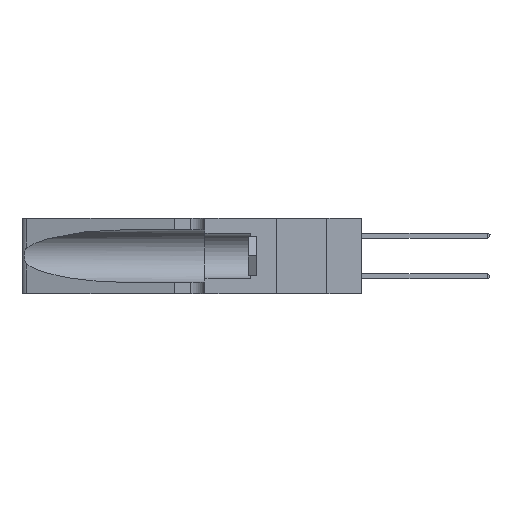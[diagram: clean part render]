
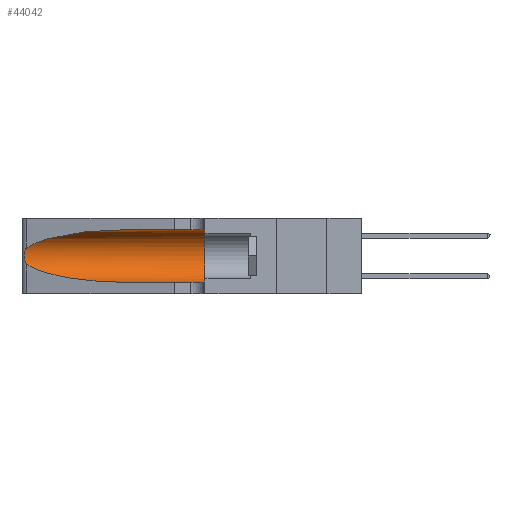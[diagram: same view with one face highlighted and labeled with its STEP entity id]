
A CAD part, left-side view. The second image highlights one B-rep face of the part: STEP entity #44042.
In plain terms, the highlighted cylindrical face has radius 3.308 mm (diameter 6.617 mm), a partial arc.
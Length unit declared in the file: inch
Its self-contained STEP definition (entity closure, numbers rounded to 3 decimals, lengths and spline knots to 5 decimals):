
#863 = CARTESIAN_POINT ( 'NONE',  ( 0.25854, 1.2359, 0.20912 ) ) ;
#1020 = CARTESIAN_POINT ( 'NONE',  ( 0.26018, 1.23835, 0.19895 ) ) ;
#1351 = DIRECTION ( 'NONE',  ( 0., -1., 0. ) ) ;
#1373 = VERTEX_POINT ( 'NONE', #34866 ) ;
#1954 = VERTEX_POINT ( 'NONE', #18898 ) ;
#2078 = DIRECTION ( 'NONE',  ( 0., -1., 0. ) ) ;
#2092 = AXIS2_PLACEMENT_3D ( 'NONE', #46518, #17487, #35357 ) ;
#2731 = CARTESIAN_POINT ( 'NONE',  ( 0.1305, 0.72297, 0.31525 ) ) ;
#3497 = CARTESIAN_POINT ( 'NONE',  ( 0.18966, 0.96281, 0.31525 ) ) ;
#3887 = ORIENTED_EDGE ( 'NONE', *, *, #15033, .T. ) ;
#4369 = CARTESIAN_POINT ( 'NONE',  ( 0.26075, 1.23896, 0.178 ) ) ;
#4590 = DIRECTION ( 'NONE',  ( 0., -1., 0. ) ) ;
#4843 = CARTESIAN_POINT ( 'NONE',  ( 0.25555, 1.22993, 0.14849 ) ) ;
#4985 = EDGE_CURVE ( 'NONE', #29005, #1954, #27852, .T. ) ;
#5172 = CARTESIAN_POINT ( 'NONE',  ( 0.1305, 1.61858, 0.185 ) ) ;
#7144 = CARTESIAN_POINT ( 'NONE',  ( 0.1305, 0.72297, 0.31525 ) ) ;
#7342 = AXIS2_PLACEMENT_3D ( 'NONE', #5172, #1351, #18997 ) ;
#7555 =( BOUNDED_CURVE ( )  B_SPLINE_CURVE ( 3, ( #23868, #20100, #12481, #26851 ),
 .UNSPECIFIED., .F., .F. ) 
 B_SPLINE_CURVE_WITH_KNOTS ( ( 4, 4 ),
 ( 3.44316, 4.71239 ),
 .UNSPECIFIED. ) 
 CURVE ( )  GEOMETRIC_REPRESENTATION_ITEM ( )  RATIONAL_B_SPLINE_CURVE ( ( 1., 0.87, 0.87, 1. ) ) 
 REPRESENTATION_ITEM ( '' )  );
#8351 = CARTESIAN_POINT ( 'NONE',  ( 0.25639, 1.23184, 0.21858 ) ) ;
#11143 = CARTESIAN_POINT ( 'NONE',  ( 0.25487, 1.22718, 0.14631 ) ) ;
#11994 = ORIENTED_EDGE ( 'NONE', *, *, #39823, .T. ) ;
#12154 = CARTESIAN_POINT ( 'NONE',  ( 0.26017, 1.23833, 0.17102 ) ) ;
#12481 = CARTESIAN_POINT ( 'NONE',  ( 0.18966, 0.96281, 0.05475 ) ) ;
#15033 = EDGE_CURVE ( 'NONE', #1954, #36051, #39171, .T. ) ;
#15307 = CARTESIAN_POINT ( 'NONE',  ( 0.25487, 1.22718, 0.22369 ) ) ;
#15538 = LINE ( 'NONE', #40557, #36487 ) ;
#16273 = CYLINDRICAL_SURFACE ( 'NONE', #7342, 0.13025 ) ;
#17487 = DIRECTION ( 'NONE',  ( 0., 1., 0. ) ) ;
#18898 = CARTESIAN_POINT ( 'NONE',  ( 0.25487, 1.22718, 0.22369 ) ) ;
#18995 = CARTESIAN_POINT ( 'NONE',  ( 0.25787, 1.23484, 0.2124 ) ) ;
#18997 = DIRECTION ( 'NONE',  ( 0., 0., -1. ) ) ;
#20015 = ORIENTED_EDGE ( 'NONE', *, *, #22002, .F. ) ;
#20100 = CARTESIAN_POINT ( 'NONE',  ( 0.2373, 1.15595, 0.08982 ) ) ;
#20306 = CARTESIAN_POINT ( 'NONE',  ( 0.1305, 0.35, 0.31525 ) ) ;
#22002 = EDGE_CURVE ( 'NONE', #40436, #1373, #23542, .T. ) ;
#22773 = EDGE_CURVE ( 'NONE', #29005, #40436, #15538, .T. ) ;
#23542 = CIRCLE ( 'NONE', #2092, 0.13025 ) ;
#23868 = CARTESIAN_POINT ( 'NONE',  ( 0.25487, 1.22718, 0.14631 ) ) ;
#24752 = FACE_OUTER_BOUND ( 'NONE', #34315, .T. ) ;
#25524 = EDGE_CURVE ( 'NONE', #36051, #34071, #7555, .T. ) ;
#26526 = CARTESIAN_POINT ( 'NONE',  ( 0.25856, 1.23593, 0.16098 ) ) ;
#26631 = ORIENTED_EDGE ( 'NONE', *, *, #25524, .T. ) ;
#26851 = CARTESIAN_POINT ( 'NONE',  ( 0.1305, 0.72297, 0.05475 ) ) ;
#27852 =( BOUNDED_CURVE ( )  B_SPLINE_CURVE ( 3, ( #7144, #3497, #28830, #39300 ),
 .UNSPECIFIED., .F., .T. ) 
 B_SPLINE_CURVE_WITH_KNOTS ( ( 4, 4 ),
 ( 1.5708, 2.84003 ),
 .UNSPECIFIED. ) 
 CURVE ( )  GEOMETRIC_REPRESENTATION_ITEM ( )  RATIONAL_B_SPLINE_CURVE ( ( 1., 0.87, 0.87, 1. ) ) 
 REPRESENTATION_ITEM ( '' )  );
#28830 = CARTESIAN_POINT ( 'NONE',  ( 0.2373, 1.15595, 0.28018 ) ) ;
#29005 = VERTEX_POINT ( 'NONE', #2731 ) ;
#29709 = CARTESIAN_POINT ( 'NONE',  ( 0.25639, 1.23186, 0.15144 ) ) ;
#30171 = CARTESIAN_POINT ( 'NONE',  ( 0.25487, 1.22718, 0.14631 ) ) ;
#33665 = CARTESIAN_POINT ( 'NONE',  ( 0.26075, 1.23896, 0.19203 ) ) ;
#33702 = LINE ( 'NONE', #38201, #42814 ) ;
#34071 = VERTEX_POINT ( 'NONE', #41200 ) ;
#34315 = EDGE_LOOP ( 'NONE', ( #35476, #3887, #26631, #11994, #20015, #35733 ) ) ;
#34866 = CARTESIAN_POINT ( 'NONE',  ( 0.1305, 0.35, 0.05475 ) ) ;
#35357 = DIRECTION ( 'NONE',  ( 0., 0., 1. ) ) ;
#35476 = ORIENTED_EDGE ( 'NONE', *, *, #4985, .T. ) ;
#35733 = ORIENTED_EDGE ( 'NONE', *, *, #22773, .F. ) ;
#36051 = VERTEX_POINT ( 'NONE', #11143 ) ;
#36487 = VECTOR ( 'NONE', #4590, 39.37008 ) ;
#38201 = CARTESIAN_POINT ( 'NONE',  ( 0.1305, 1.61858, 0.05475 ) ) ;
#39171 = B_SPLINE_CURVE_WITH_KNOTS ( 'NONE', 3,
 ( #15307, #40816, #8351, #18995, #863, #1020, #33665, #4369, #12154, #26526, #40653, #29709, #4843, #30171 ),
 .UNSPECIFIED., .F., .F.,
 ( 4, 2, 2, 2, 2, 2, 4 ),
 ( 0., 0.00027, 0.00053, 0.00107, 0.0016, 0.00187, 0.00214 ),
 .UNSPECIFIED. ) ;
#39300 = CARTESIAN_POINT ( 'NONE',  ( 0.25487, 1.22718, 0.22369 ) ) ;
#39823 = EDGE_CURVE ( 'NONE', #34071, #1373, #33702, .T. ) ;
#40436 = VERTEX_POINT ( 'NONE', #20306 ) ;
#40557 = CARTESIAN_POINT ( 'NONE',  ( 0.1305, 1.61858, 0.31525 ) ) ;
#40653 = CARTESIAN_POINT ( 'NONE',  ( 0.25789, 1.23486, 0.15765 ) ) ;
#40816 = CARTESIAN_POINT ( 'NONE',  ( 0.25555, 1.22994, 0.2215 ) ) ;
#41200 = CARTESIAN_POINT ( 'NONE',  ( 0.1305, 0.72297, 0.05475 ) ) ;
#42814 = VECTOR ( 'NONE', #2078, 39.37008 ) ;
#44042 = ADVANCED_FACE ( 'NONE', ( #24752 ), #16273, .F. ) ;
#46518 = CARTESIAN_POINT ( 'NONE',  ( 0.1305, 0.35, 0.185 ) ) ;
